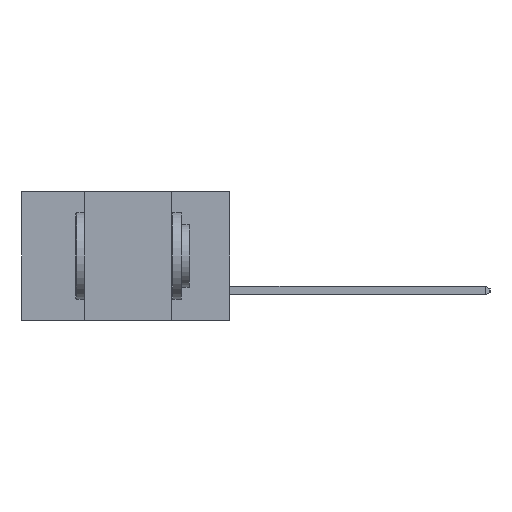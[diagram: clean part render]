
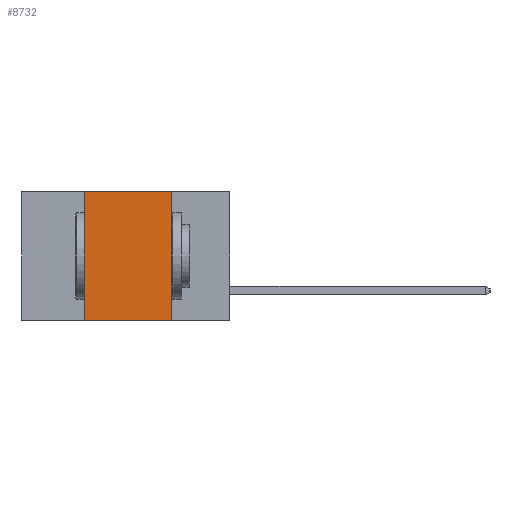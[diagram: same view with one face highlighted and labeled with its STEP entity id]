
A CAD part, left-side view. The second image highlights one B-rep face of the part: STEP entity #8732.
In plain terms, the highlighted planar face has unit normal (-1, 0, 0).
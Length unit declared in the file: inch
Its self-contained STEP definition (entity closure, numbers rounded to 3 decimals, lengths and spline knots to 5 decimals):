
#362 = EDGE_CURVE ( 'NONE', #7354, #7918, #10439, .T. ) ;
#1353 = LINE ( 'NONE', #15034, #5692 ) ;
#1636 = VECTOR ( 'NONE', #22141, 39.37008 ) ;
#2384 = EDGE_CURVE ( 'NONE', #10672, #20417, #1353, .T. ) ;
#2485 = EDGE_LOOP ( 'NONE', ( #12414, #3173, #8789, #15056 ) ) ;
#3149 = CARTESIAN_POINT ( 'NONE',  ( 0., 0.42, 0. ) ) ;
#3173 = ORIENTED_EDGE ( 'NONE', *, *, #2384, .F. ) ;
#3377 = CARTESIAN_POINT ( 'NONE',  ( 0., 0.42, -0.37 ) ) ;
#5273 = CARTESIAN_POINT ( 'NONE',  ( 0., 0.17, 0. ) ) ;
#5437 = CARTESIAN_POINT ( 'NONE',  ( 0., 0.17, -0.37 ) ) ;
#5692 = VECTOR ( 'NONE', #15166, 39.37008 ) ;
#7354 = VERTEX_POINT ( 'NONE', #3377 ) ;
#7815 = CARTESIAN_POINT ( 'NONE',  ( 0., 0.17, -0.37 ) ) ;
#7918 = VERTEX_POINT ( 'NONE', #5437 ) ;
#8732 = ADVANCED_FACE ( 'NONE', ( #24524 ), #14091, .F. ) ;
#8789 = ORIENTED_EDGE ( 'NONE', *, *, #23624, .F. ) ;
#8797 = DIRECTION ( 'NONE',  ( 0., -1., 0. ) ) ;
#10439 = LINE ( 'NONE', #14691, #25966 ) ;
#10672 = VERTEX_POINT ( 'NONE', #3149 ) ;
#10926 = VECTOR ( 'NONE', #12974, 39.37008 ) ;
#12256 = LINE ( 'NONE', #7815, #1636 ) ;
#12414 = ORIENTED_EDGE ( 'NONE', *, *, #14243, .F. ) ;
#12974 = DIRECTION ( 'NONE',  ( 0., 0., 1. ) ) ;
#14001 = DIRECTION ( 'NONE',  ( 0., 0., -1. ) ) ;
#14091 = PLANE ( 'NONE',  #25138 ) ;
#14127 = DIRECTION ( 'NONE',  ( 1., 0., 0. ) ) ;
#14243 = EDGE_CURVE ( 'NONE', #20417, #7918, #12256, .T. ) ;
#14657 = CARTESIAN_POINT ( 'NONE',  ( 0., 0.6, 0. ) ) ;
#14691 = CARTESIAN_POINT ( 'NONE',  ( 0., 0.6, -0.37 ) ) ;
#15034 = CARTESIAN_POINT ( 'NONE',  ( 0., 0.6, 0. ) ) ;
#15056 = ORIENTED_EDGE ( 'NONE', *, *, #362, .T. ) ;
#15166 = DIRECTION ( 'NONE',  ( 0., -1., 0. ) ) ;
#20417 = VERTEX_POINT ( 'NONE', #5273 ) ;
#22141 = DIRECTION ( 'NONE',  ( 0., 0., -1. ) ) ;
#23624 = EDGE_CURVE ( 'NONE', #7354, #10672, #26416, .T. ) ;
#24524 = FACE_OUTER_BOUND ( 'NONE', #2485, .T. ) ;
#25032 = CARTESIAN_POINT ( 'NONE',  ( 0., 0.42, -0.37 ) ) ;
#25138 = AXIS2_PLACEMENT_3D ( 'NONE', #14657, #14127, #14001 ) ;
#25966 = VECTOR ( 'NONE', #8797, 39.37008 ) ;
#26416 = LINE ( 'NONE', #25032, #10926 ) ;
